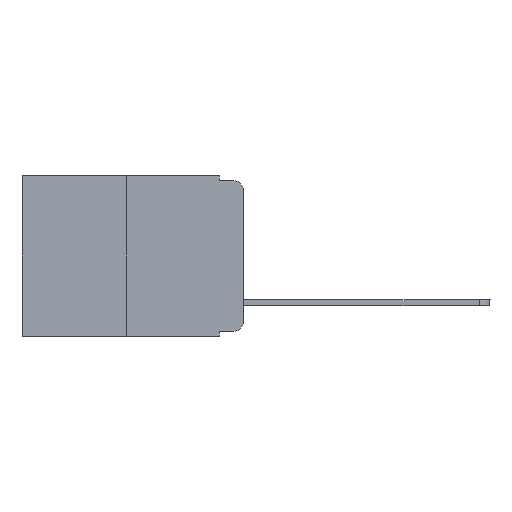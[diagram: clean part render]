
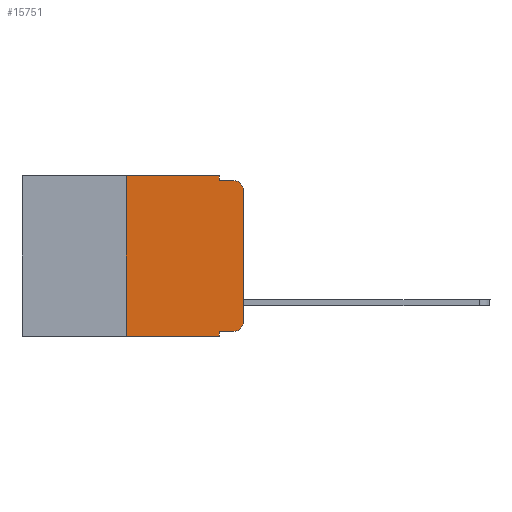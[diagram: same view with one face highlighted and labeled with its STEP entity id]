
A CAD part, left-side view. The second image highlights one B-rep face of the part: STEP entity #15751.
In plain terms, the highlighted planar face has unit normal (-1, 0, 0).
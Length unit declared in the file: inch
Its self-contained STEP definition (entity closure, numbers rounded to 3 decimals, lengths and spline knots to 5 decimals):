
#65 = LINE ( 'NONE', #17470, #12266 ) ;
#197 = ORIENTED_EDGE ( 'NONE', *, *, #11881, .T. ) ;
#230 = EDGE_CURVE ( 'NONE', #19923, #8677, #18366, .T. ) ;
#342 = CARTESIAN_POINT ( 'NONE',  ( 0., 0.051, -0.01 ) ) ;
#472 = VECTOR ( 'NONE', #20014, 39.37008 ) ;
#574 = VERTEX_POINT ( 'NONE', #4404 ) ;
#740 = VECTOR ( 'NONE', #17802, 39.37008 ) ;
#1106 = CARTESIAN_POINT ( 'NONE',  ( 0., 0.473, 0. ) ) ;
#1516 = ORIENTED_EDGE ( 'NONE', *, *, #4888, .F. ) ;
#1733 = EDGE_CURVE ( 'NONE', #7704, #9695, #10707, .T. ) ;
#1948 = EDGE_CURVE ( 'NONE', #19923, #13753, #17805, .T. ) ;
#2179 = CARTESIAN_POINT ( 'NONE',  ( 0., 0.051, -0.343 ) ) ;
#2577 = DIRECTION ( 'NONE',  ( 0., 0., -1. ) ) ;
#2898 = CARTESIAN_POINT ( 'NONE',  ( 0., 0.051, -0.333 ) ) ;
#2982 = VECTOR ( 'NONE', #10568, 39.37008 ) ;
#3345 = VECTOR ( 'NONE', #8110, 39.37008 ) ;
#3435 = ORIENTED_EDGE ( 'NONE', *, *, #1948, .T. ) ;
#3563 = AXIS2_PLACEMENT_3D ( 'NONE', #5951, #6165, #14059 ) ;
#3646 = AXIS2_PLACEMENT_3D ( 'NONE', #1106, #12337, #10577 ) ;
#3698 = VERTEX_POINT ( 'NONE', #342 ) ;
#4120 = CARTESIAN_POINT ( 'NONE',  ( 0., 0.02, -0.01 ) ) ;
#4135 = CARTESIAN_POINT ( 'NONE',  ( 0., 0.02, -0.03 ) ) ;
#4387 = ORIENTED_EDGE ( 'NONE', *, *, #8689, .F. ) ;
#4404 = CARTESIAN_POINT ( 'NONE',  ( 0., 0., -0.03 ) ) ;
#4553 = CARTESIAN_POINT ( 'NONE',  ( 0., 0.051, -0.01 ) ) ;
#4888 = EDGE_CURVE ( 'NONE', #14692, #3698, #12294, .T. ) ;
#5164 = DIRECTION ( 'NONE',  ( 0., -1., 0. ) ) ;
#5240 = CARTESIAN_POINT ( 'NONE',  ( 0., 0.473, 0. ) ) ;
#5951 = CARTESIAN_POINT ( 'NONE',  ( 0., 0.02, -0.313 ) ) ;
#6165 = DIRECTION ( 'NONE',  ( -1., 0., 0. ) ) ;
#6368 = EDGE_LOOP ( 'NONE', ( #197, #17444, #8817, #1516, #13691, #6672, #3435, #4387, #13616, #8994 ) ) ;
#6672 = ORIENTED_EDGE ( 'NONE', *, *, #230, .F. ) ;
#7373 = CARTESIAN_POINT ( 'NONE',  ( 0., 0.051, 0. ) ) ;
#7405 = DIRECTION ( 'NONE',  ( 0., 0., -1. ) ) ;
#7546 = DIRECTION ( 'NONE',  ( -1., 0., 0. ) ) ;
#7704 = VERTEX_POINT ( 'NONE', #11106 ) ;
#8110 = DIRECTION ( 'NONE',  ( 0., 0., 1. ) ) ;
#8677 = VERTEX_POINT ( 'NONE', #19507 ) ;
#8689 = EDGE_CURVE ( 'NONE', #17147, #13753, #12667, .T. ) ;
#8738 = VECTOR ( 'NONE', #2577, 39.37008 ) ;
#8817 = ORIENTED_EDGE ( 'NONE', *, *, #13415, .F. ) ;
#8853 = EDGE_CURVE ( 'NONE', #8677, #14692, #16742, .T. ) ;
#8994 = ORIENTED_EDGE ( 'NONE', *, *, #1733, .T. ) ;
#9040 = VECTOR ( 'NONE', #16069, 39.37008 ) ;
#9229 = CARTESIAN_POINT ( 'NONE',  ( 0., 0.25, -0.343 ) ) ;
#9695 = VERTEX_POINT ( 'NONE', #17275 ) ;
#10568 = DIRECTION ( 'NONE',  ( 0., -1., 0. ) ) ;
#10577 = DIRECTION ( 'NONE',  ( 0., 0., -1. ) ) ;
#10707 = CIRCLE ( 'NONE', #3563, 0.02 ) ;
#11036 = CARTESIAN_POINT ( 'NONE',  ( 0., 0.051, 0. ) ) ;
#11106 = CARTESIAN_POINT ( 'NONE',  ( 0., 0.02, -0.333 ) ) ;
#11881 = EDGE_CURVE ( 'NONE', #9695, #574, #15485, .T. ) ;
#12088 = VERTEX_POINT ( 'NONE', #4120 ) ;
#12266 = VECTOR ( 'NONE', #12505, 39.37008 ) ;
#12271 = PLANE ( 'NONE',  #3646 ) ;
#12294 = LINE ( 'NONE', #7373, #8738 ) ;
#12337 = DIRECTION ( 'NONE',  ( 1., 0., 0. ) ) ;
#12505 = DIRECTION ( 'NONE',  ( 0., -1., 0. ) ) ;
#12667 = LINE ( 'NONE', #19428, #740 ) ;
#13009 = FACE_OUTER_BOUND ( 'NONE', #6368, .T. ) ;
#13415 = EDGE_CURVE ( 'NONE', #3698, #12088, #15153, .T. ) ;
#13490 = VECTOR ( 'NONE', #5164, 39.37008 ) ;
#13616 = ORIENTED_EDGE ( 'NONE', *, *, #19875, .T. ) ;
#13627 = AXIS2_PLACEMENT_3D ( 'NONE', #4135, #7546, #7405 ) ;
#13691 = ORIENTED_EDGE ( 'NONE', *, *, #8853, .F. ) ;
#13753 = VERTEX_POINT ( 'NONE', #2179 ) ;
#14059 = DIRECTION ( 'NONE',  ( 0., 0., -1. ) ) ;
#14692 = VERTEX_POINT ( 'NONE', #11036 ) ;
#14880 = CARTESIAN_POINT ( 'NONE',  ( 0., 0.25, 0. ) ) ;
#15153 = LINE ( 'NONE', #4553, #9040 ) ;
#15485 = LINE ( 'NONE', #16638, #472 ) ;
#15751 = ADVANCED_FACE ( 'NONE', ( #13009 ), #12271, .F. ) ;
#16069 = DIRECTION ( 'NONE',  ( 0., -1., 0. ) ) ;
#16115 = CARTESIAN_POINT ( 'NONE',  ( 0., 0.473, -0.343 ) ) ;
#16638 = CARTESIAN_POINT ( 'NONE',  ( 0., 0., 0. ) ) ;
#16742 = LINE ( 'NONE', #5240, #2982 ) ;
#17147 = VERTEX_POINT ( 'NONE', #2898 ) ;
#17275 = CARTESIAN_POINT ( 'NONE',  ( 0., 0., -0.313 ) ) ;
#17444 = ORIENTED_EDGE ( 'NONE', *, *, #19812, .T. ) ;
#17470 = CARTESIAN_POINT ( 'NONE',  ( 0., 0.051, -0.333 ) ) ;
#17802 = DIRECTION ( 'NONE',  ( 0., 0., -1. ) ) ;
#17805 = LINE ( 'NONE', #16115, #13490 ) ;
#18366 = LINE ( 'NONE', #14880, #3345 ) ;
#19120 = CIRCLE ( 'NONE', #13627, 0.02 ) ;
#19428 = CARTESIAN_POINT ( 'NONE',  ( 0., 0.051, 0. ) ) ;
#19507 = CARTESIAN_POINT ( 'NONE',  ( 0., 0.25, 0. ) ) ;
#19812 = EDGE_CURVE ( 'NONE', #574, #12088, #19120, .T. ) ;
#19875 = EDGE_CURVE ( 'NONE', #17147, #7704, #65, .T. ) ;
#19923 = VERTEX_POINT ( 'NONE', #9229 ) ;
#20014 = DIRECTION ( 'NONE',  ( 0., 0., 1. ) ) ;
